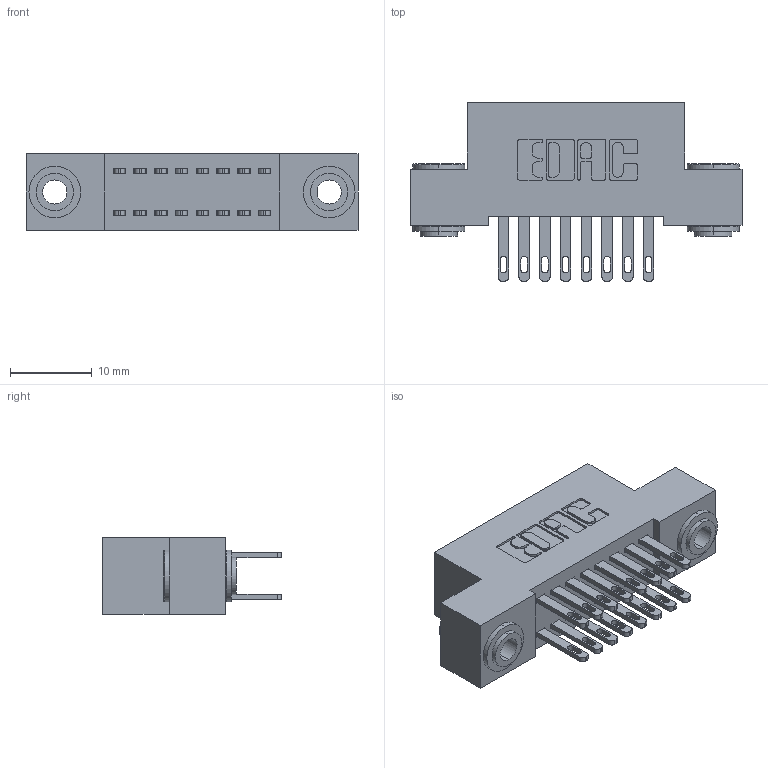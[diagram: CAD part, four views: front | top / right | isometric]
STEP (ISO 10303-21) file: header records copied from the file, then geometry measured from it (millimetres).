
FILE_DESCRIPTION (( 'STEP AP203' ), '1' );
FILE_NAME ('892-016-500-203.STEP', '2020-09-21T13:30:08', ( '' ), ( '' ), 'SwSTEP 2.0', 'SolidWorks 2020', '' );
FILE_SCHEMA (( 'CONFIG_CONTROL_DESIGN' ));
Length unit declared in the file: inch
Products named in the file (4): 345-292-001_345-293-100; 892-016-500-203; 842 Part_.156 TH; 342-250-002_345-250-002-102
Assembly tree (19 placements, depth 2):
  892-016-500-203
    842 Part_.156 TH
    345-292-001_345-293-100  x16
    342-250-002_345-250-002-102  x2
Bounding box: 40.64 x 21.85 x 9.4 mm (x, y, z)
Volume: 3562.3 mm3; surface area: 5328 mm2
Topology: 19 solids, 19 shells, 916 faces, 2727 edges, 1814 vertices
Faces by surface type: plane 556, cylinder 352, cone 8
Entity records: 9992 total; most frequent: CARTESIAN_POINT 1669, ORIENTED_EDGE 1598, DIRECTION 1521, EDGE_CURVE 799, VECTOR 643, LINE 643, VERTEX_POINT 530, AXIS2_PLACEMENT_3D 439
